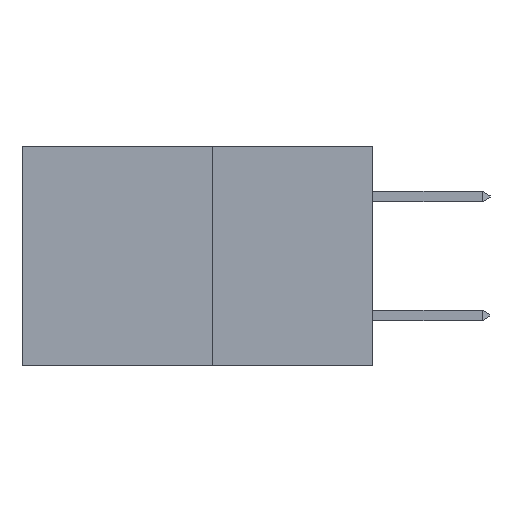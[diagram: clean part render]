
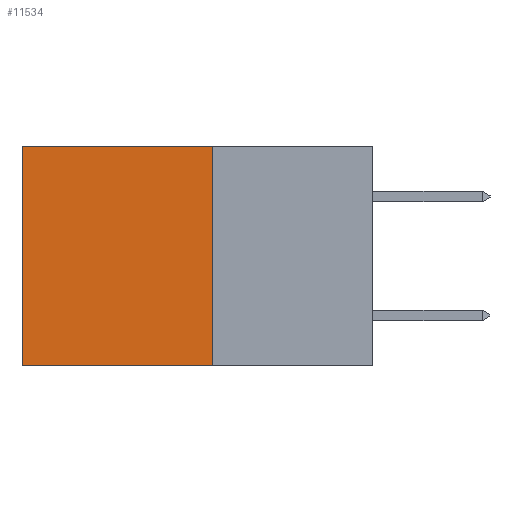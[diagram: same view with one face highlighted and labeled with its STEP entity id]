
A CAD part, left-side view. The second image highlights one B-rep face of the part: STEP entity #11534.
In plain terms, the highlighted planar face has unit normal (-1, 0, 0).
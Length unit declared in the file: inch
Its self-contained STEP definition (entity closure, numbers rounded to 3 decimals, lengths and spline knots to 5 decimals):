
#62 = DIRECTION ( 'NONE',  ( 1., 0., 0. ) ) ;
#484 = EDGE_LOOP ( 'NONE', ( #1645, #15814, #13722, #6249 ) ) ;
#1645 = ORIENTED_EDGE ( 'NONE', *, *, #17334, .T. ) ;
#2214 = CARTESIAN_POINT ( 'NONE',  ( 0.277, 0.59, -0.37 ) ) ;
#2527 = CARTESIAN_POINT ( 'NONE',  ( 0.277, 0.59, 0. ) ) ;
#2557 = VERTEX_POINT ( 'NONE', #2214 ) ;
#3062 = FACE_OUTER_BOUND ( 'NONE', #484, .T. ) ;
#3382 = VERTEX_POINT ( 'NONE', #2527 ) ;
#3965 = DIRECTION ( 'NONE',  ( 0., 1., 0. ) ) ;
#4018 = CARTESIAN_POINT ( 'NONE',  ( 0.277, 0.27, 0. ) ) ;
#4133 = VECTOR ( 'NONE', #8962, 39.37008 ) ;
#4245 = EDGE_CURVE ( 'NONE', #13737, #2557, #13970, .T. ) ;
#4787 = EDGE_CURVE ( 'NONE', #14726, #3382, #16156, .T. ) ;
#6249 = ORIENTED_EDGE ( 'NONE', *, *, #4787, .T. ) ;
#7640 = CARTESIAN_POINT ( 'NONE',  ( 0.277, 0.59, -0.37 ) ) ;
#8855 = AXIS2_PLACEMENT_3D ( 'NONE', #13615, #62, #9585 ) ;
#8962 = DIRECTION ( 'NONE',  ( 0., 0., -1. ) ) ;
#8992 = CARTESIAN_POINT ( 'NONE',  ( 0.277, 0.27, -0.37 ) ) ;
#9532 = VECTOR ( 'NONE', #9843, 39.37008 ) ;
#9585 = DIRECTION ( 'NONE',  ( 0., 0., -1. ) ) ;
#9744 = CARTESIAN_POINT ( 'NONE',  ( 0.277, 0.27, -0.37 ) ) ;
#9843 = DIRECTION ( 'NONE',  ( 0., 1., 0. ) ) ;
#10392 = DIRECTION ( 'NONE',  ( 0., 0., -1. ) ) ;
#10593 = EDGE_CURVE ( 'NONE', #14726, #13737, #13314, .T. ) ;
#11262 = LINE ( 'NONE', #7640, #4133 ) ;
#11534 = ADVANCED_FACE ( 'NONE', ( #3062 ), #16196, .F. ) ;
#12333 = VECTOR ( 'NONE', #3965, 39.37008 ) ;
#13314 = LINE ( 'NONE', #8992, #16322 ) ;
#13615 = CARTESIAN_POINT ( 'NONE',  ( 0.277, 0.27, -0.37 ) ) ;
#13722 = ORIENTED_EDGE ( 'NONE', *, *, #10593, .F. ) ;
#13737 = VERTEX_POINT ( 'NONE', #17375 ) ;
#13970 = LINE ( 'NONE', #9744, #9532 ) ;
#14726 = VERTEX_POINT ( 'NONE', #16447 ) ;
#15814 = ORIENTED_EDGE ( 'NONE', *, *, #4245, .F. ) ;
#16156 = LINE ( 'NONE', #4018, #12333 ) ;
#16196 = PLANE ( 'NONE',  #8855 ) ;
#16322 = VECTOR ( 'NONE', #10392, 39.37008 ) ;
#16447 = CARTESIAN_POINT ( 'NONE',  ( 0.277, 0.27, 0. ) ) ;
#17334 = EDGE_CURVE ( 'NONE', #3382, #2557, #11262, .T. ) ;
#17375 = CARTESIAN_POINT ( 'NONE',  ( 0.277, 0.27, -0.37 ) ) ;
